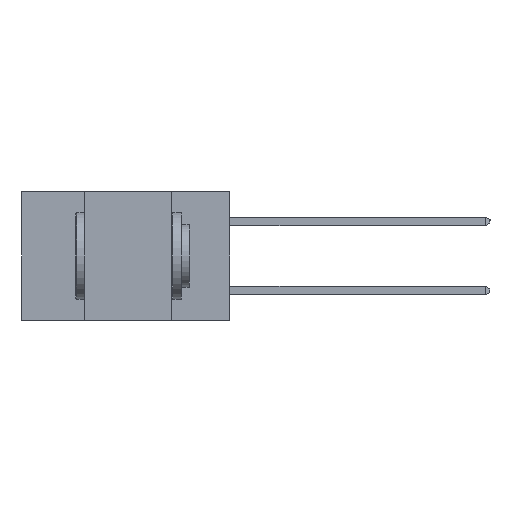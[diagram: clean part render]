
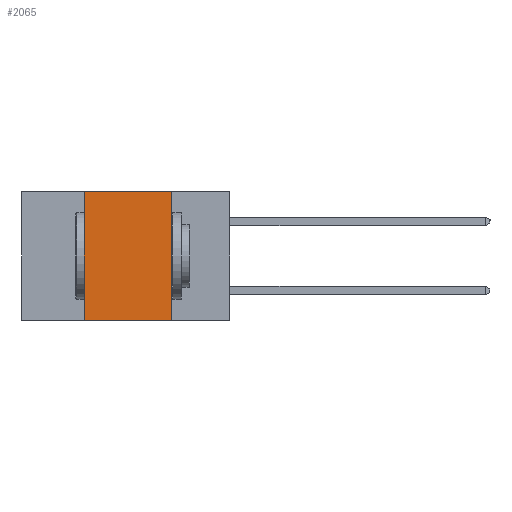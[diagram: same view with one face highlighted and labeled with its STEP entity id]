
A CAD part, left-side view. The second image highlights one B-rep face of the part: STEP entity #2065.
In plain terms, the highlighted planar face has unit normal (-1, 0, 0).
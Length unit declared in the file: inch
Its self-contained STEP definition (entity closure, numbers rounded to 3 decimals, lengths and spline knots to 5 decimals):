
#156 = ORIENTED_EDGE ( 'NONE', *, *, #9543, .F. ) ;
#646 = VECTOR ( 'NONE', #11082, 39.37008 ) ;
#950 = DIRECTION ( 'NONE',  ( 0., -1., 0. ) ) ;
#1064 = CARTESIAN_POINT ( 'NONE',  ( 0., 0.42, -0.37 ) ) ;
#1148 = VERTEX_POINT ( 'NONE', #1064 ) ;
#1324 = VERTEX_POINT ( 'NONE', #11317 ) ;
#1795 = VECTOR ( 'NONE', #2745, 39.37008 ) ;
#2065 = ADVANCED_FACE ( 'NONE', ( #7239 ), #4333, .F. ) ;
#2220 = CARTESIAN_POINT ( 'NONE',  ( 0., 0.6, 0. ) ) ;
#2677 = VECTOR ( 'NONE', #15316, 39.37008 ) ;
#2745 = DIRECTION ( 'NONE',  ( 0., 0., -1. ) ) ;
#3068 = EDGE_CURVE ( 'NONE', #1148, #11069, #4517, .T. ) ;
#4333 = PLANE ( 'NONE',  #12724 ) ;
#4517 = LINE ( 'NONE', #9576, #13779 ) ;
#5126 = EDGE_CURVE ( 'NONE', #1148, #1324, #13030, .T. ) ;
#7239 = FACE_OUTER_BOUND ( 'NONE', #9218, .T. ) ;
#7733 = LINE ( 'NONE', #7806, #1795 ) ;
#7806 = CARTESIAN_POINT ( 'NONE',  ( 0., 0.17, -0.37 ) ) ;
#7906 = VERTEX_POINT ( 'NONE', #12002 ) ;
#8118 = DIRECTION ( 'NONE',  ( 0., 0., -1. ) ) ;
#8914 = ORIENTED_EDGE ( 'NONE', *, *, #3068, .T. ) ;
#9218 = EDGE_LOOP ( 'NONE', ( #156, #10680, #10496, #8914 ) ) ;
#9392 = CARTESIAN_POINT ( 'NONE',  ( 0., 0.6, 0. ) ) ;
#9543 = EDGE_CURVE ( 'NONE', #7906, #11069, #7733, .T. ) ;
#9576 = CARTESIAN_POINT ( 'NONE',  ( 0., 0.6, -0.37 ) ) ;
#10496 = ORIENTED_EDGE ( 'NONE', *, *, #5126, .F. ) ;
#10680 = ORIENTED_EDGE ( 'NONE', *, *, #13237, .F. ) ;
#11069 = VERTEX_POINT ( 'NONE', #12842 ) ;
#11082 = DIRECTION ( 'NONE',  ( 0., -1., 0. ) ) ;
#11317 = CARTESIAN_POINT ( 'NONE',  ( 0., 0.42, 0. ) ) ;
#11456 = CARTESIAN_POINT ( 'NONE',  ( 0., 0.42, -0.37 ) ) ;
#12002 = CARTESIAN_POINT ( 'NONE',  ( 0., 0.17, 0. ) ) ;
#12724 = AXIS2_PLACEMENT_3D ( 'NONE', #9392, #14424, #8118 ) ;
#12842 = CARTESIAN_POINT ( 'NONE',  ( 0., 0.17, -0.37 ) ) ;
#13030 = LINE ( 'NONE', #11456, #2677 ) ;
#13237 = EDGE_CURVE ( 'NONE', #1324, #7906, #13565, .T. ) ;
#13565 = LINE ( 'NONE', #2220, #646 ) ;
#13779 = VECTOR ( 'NONE', #950, 39.37008 ) ;
#14424 = DIRECTION ( 'NONE',  ( 1., 0., 0. ) ) ;
#15316 = DIRECTION ( 'NONE',  ( 0., 0., 1. ) ) ;
